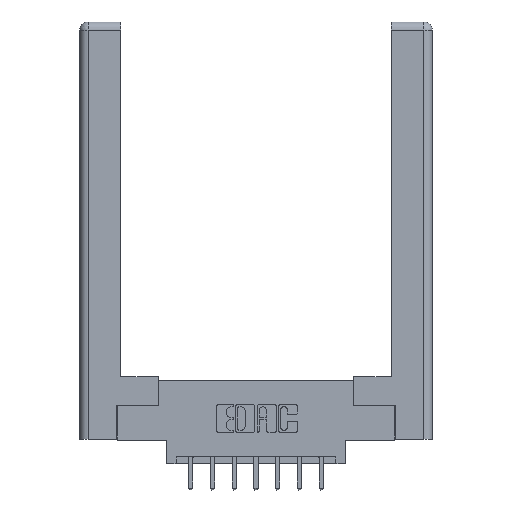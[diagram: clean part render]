
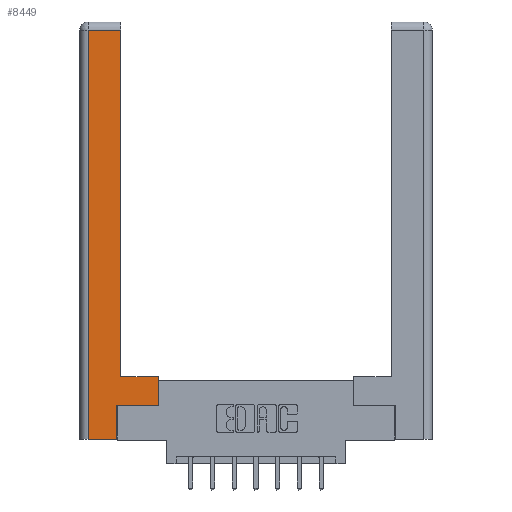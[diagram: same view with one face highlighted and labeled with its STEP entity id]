
A CAD part, top view. The second image highlights one B-rep face of the part: STEP entity #8449.
In plain terms, the highlighted planar face has unit normal (0, 0, 1).
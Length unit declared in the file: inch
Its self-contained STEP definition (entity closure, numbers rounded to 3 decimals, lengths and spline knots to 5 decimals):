
#28 = VECTOR ( 'NONE', #2849, 39.37008 ) ;
#39 = DIRECTION ( 'NONE',  ( 0., 1., 0. ) ) ;
#69 = VECTOR ( 'NONE', #593, 39.37008 ) ;
#593 = DIRECTION ( 'NONE',  ( 0., 1., 0. ) ) ;
#654 = LINE ( 'NONE', #5298, #9356 ) ;
#764 = VECTOR ( 'NONE', #4849, 39.37008 ) ;
#854 = VECTOR ( 'NONE', #39, 39.37008 ) ;
#1048 = CARTESIAN_POINT ( 'NONE',  ( 0.265, 0.245, 0. ) ) ;
#1144 = EDGE_CURVE ( 'NONE', #9876, #11128, #654, .T. ) ;
#1269 = EDGE_CURVE ( 'NONE', #10112, #6310, #7176, .T. ) ;
#1317 = DIRECTION ( 'NONE',  ( 0., 1., 0. ) ) ;
#1366 = CARTESIAN_POINT ( 'NONE',  ( 0.565, 0.45, 0. ) ) ;
#1795 = VECTOR ( 'NONE', #6549, 39.37008 ) ;
#1851 = ORIENTED_EDGE ( 'NONE', *, *, #9388, .T. ) ;
#2118 = ORIENTED_EDGE ( 'NONE', *, *, #8034, .T. ) ;
#2516 = PLANE ( 'NONE',  #5692 ) ;
#2715 = DIRECTION ( 'NONE',  ( 1., 0., 0. ) ) ;
#2849 = DIRECTION ( 'NONE',  ( -1., 0., 0. ) ) ;
#3458 = CARTESIAN_POINT ( 'NONE',  ( 0.295, 2.94, 0. ) ) ;
#3643 = CARTESIAN_POINT ( 'NONE',  ( 0., 0., 0. ) ) ;
#3719 = CARTESIAN_POINT ( 'NONE',  ( 0.265, 0., 0. ) ) ;
#4431 = EDGE_LOOP ( 'NONE', ( #4516, #10510, #2118, #6514, #12714, #1851, #9615, #11145 ) ) ;
#4434 = CARTESIAN_POINT ( 'NONE',  ( 0.0615, 2.94, 0. ) ) ;
#4516 = ORIENTED_EDGE ( 'NONE', *, *, #5600, .T. ) ;
#4701 = CARTESIAN_POINT ( 'NONE',  ( 0.0615, 2.94, 0. ) ) ;
#4800 = VERTEX_POINT ( 'NONE', #9150 ) ;
#4823 = CARTESIAN_POINT ( 'NONE',  ( 0.295, 0.45, 0. ) ) ;
#4849 = DIRECTION ( 'NONE',  ( 0., -1., 0. ) ) ;
#5078 = EDGE_CURVE ( 'NONE', #4800, #10112, #9085, .T. ) ;
#5092 = LINE ( 'NONE', #4434, #7093 ) ;
#5298 = CARTESIAN_POINT ( 'NONE',  ( 0.265, 0.245, 0. ) ) ;
#5528 = EDGE_CURVE ( 'NONE', #8258, #9876, #11419, .T. ) ;
#5600 = EDGE_CURVE ( 'NONE', #6310, #7394, #9237, .T. ) ;
#5655 = VECTOR ( 'NONE', #2715, 39.37008 ) ;
#5692 = AXIS2_PLACEMENT_3D ( 'NONE', #3643, #8575, #8486 ) ;
#6310 = VERTEX_POINT ( 'NONE', #9308 ) ;
#6514 = ORIENTED_EDGE ( 'NONE', *, *, #5528, .T. ) ;
#6549 = DIRECTION ( 'NONE',  ( 1., 0., 0. ) ) ;
#6698 = CARTESIAN_POINT ( 'NONE',  ( 0.265, 0., 0. ) ) ;
#7093 = VECTOR ( 'NONE', #12455, 39.37008 ) ;
#7176 = LINE ( 'NONE', #4823, #28 ) ;
#7394 = VERTEX_POINT ( 'NONE', #3458 ) ;
#8034 = EDGE_CURVE ( 'NONE', #12285, #8258, #8686, .T. ) ;
#8258 = VERTEX_POINT ( 'NONE', #10068 ) ;
#8449 = ADVANCED_FACE ( 'NONE', ( #12686 ), #2516, .F. ) ;
#8486 = DIRECTION ( 'NONE',  ( -1., 0., 0. ) ) ;
#8515 = EDGE_CURVE ( 'NONE', #7394, #12285, #5092, .T. ) ;
#8575 = DIRECTION ( 'NONE',  ( 0., 0., -1. ) ) ;
#8686 = LINE ( 'NONE', #8889, #764 ) ;
#8889 = CARTESIAN_POINT ( 'NONE',  ( 0.0615, 0., 0. ) ) ;
#9085 = LINE ( 'NONE', #11494, #69 ) ;
#9150 = CARTESIAN_POINT ( 'NONE',  ( 0.565, 0.245, 0. ) ) ;
#9237 = LINE ( 'NONE', #11979, #854 ) ;
#9274 = LINE ( 'NONE', #11467, #1795 ) ;
#9308 = CARTESIAN_POINT ( 'NONE',  ( 0.295, 0.45, 0. ) ) ;
#9356 = VECTOR ( 'NONE', #1317, 39.37008 ) ;
#9388 = EDGE_CURVE ( 'NONE', #11128, #4800, #9274, .T. ) ;
#9615 = ORIENTED_EDGE ( 'NONE', *, *, #5078, .T. ) ;
#9876 = VERTEX_POINT ( 'NONE', #6698 ) ;
#10068 = CARTESIAN_POINT ( 'NONE',  ( 0.0615, 0., 0. ) ) ;
#10112 = VERTEX_POINT ( 'NONE', #1366 ) ;
#10510 = ORIENTED_EDGE ( 'NONE', *, *, #8515, .T. ) ;
#11128 = VERTEX_POINT ( 'NONE', #1048 ) ;
#11145 = ORIENTED_EDGE ( 'NONE', *, *, #1269, .T. ) ;
#11419 = LINE ( 'NONE', #3719, #5655 ) ;
#11467 = CARTESIAN_POINT ( 'NONE',  ( 0.565, 0.245, 0. ) ) ;
#11494 = CARTESIAN_POINT ( 'NONE',  ( 0.565, 0.45, 0. ) ) ;
#11979 = CARTESIAN_POINT ( 'NONE',  ( 0.295, 3., 0. ) ) ;
#12285 = VERTEX_POINT ( 'NONE', #4701 ) ;
#12455 = DIRECTION ( 'NONE',  ( -1., 0., 0. ) ) ;
#12686 = FACE_OUTER_BOUND ( 'NONE', #4431, .T. ) ;
#12714 = ORIENTED_EDGE ( 'NONE', *, *, #1144, .T. ) ;
